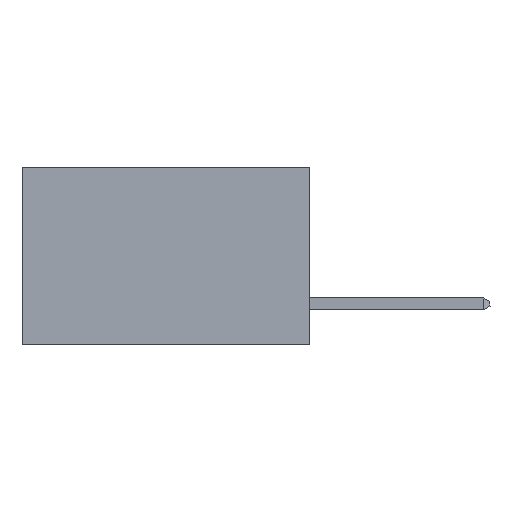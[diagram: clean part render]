
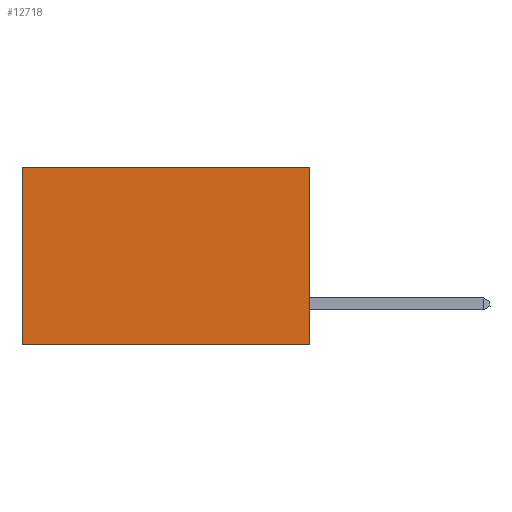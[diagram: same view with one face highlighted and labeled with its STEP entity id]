
A CAD part, left-side view. The second image highlights one B-rep face of the part: STEP entity #12718.
In plain terms, the highlighted planar face has unit normal (-1, 0, 0).
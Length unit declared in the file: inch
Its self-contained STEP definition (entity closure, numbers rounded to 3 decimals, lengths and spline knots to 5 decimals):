
#42 = DIRECTION ( 'NONE',  ( 0., 1., 0. ) ) ;
#250 = LINE ( 'NONE', #8095, #5584 ) ;
#330 = DIRECTION ( 'NONE',  ( 0., 0., -1. ) ) ;
#371 = VERTEX_POINT ( 'NONE', #1072 ) ;
#444 = VECTOR ( 'NONE', #42, 39.37008 ) ;
#823 = LINE ( 'NONE', #10963, #444 ) ;
#824 = DIRECTION ( 'NONE',  ( 1., 0., 0. ) ) ;
#1034 = VECTOR ( 'NONE', #9453, 39.37008 ) ;
#1072 = CARTESIAN_POINT ( 'NONE',  ( 0.2875, 0.6, -0.37 ) ) ;
#1482 = ORIENTED_EDGE ( 'NONE', *, *, #14352, .F. ) ;
#1924 = CARTESIAN_POINT ( 'NONE',  ( 0.2875, 0., 0. ) ) ;
#2628 = AXIS2_PLACEMENT_3D ( 'NONE', #1924, #824, #11736 ) ;
#2763 = CARTESIAN_POINT ( 'NONE',  ( 0.2875, 0., 0. ) ) ;
#3373 = EDGE_CURVE ( 'NONE', #14773, #12495, #250, .T. ) ;
#3547 = LINE ( 'NONE', #10750, #1034 ) ;
#3920 = ORIENTED_EDGE ( 'NONE', *, *, #14530, .F. ) ;
#4230 = CARTESIAN_POINT ( 'NONE',  ( 0.2875, 0., -0.37 ) ) ;
#4263 = VERTEX_POINT ( 'NONE', #4230 ) ;
#4431 = PLANE ( 'NONE',  #2628 ) ;
#5317 = LINE ( 'NONE', #15131, #14573 ) ;
#5584 = VECTOR ( 'NONE', #9321, 39.37008 ) ;
#5759 = CARTESIAN_POINT ( 'NONE',  ( 0.2875, 0.6, 0. ) ) ;
#7109 = ORIENTED_EDGE ( 'NONE', *, *, #3373, .T. ) ;
#8095 = CARTESIAN_POINT ( 'NONE',  ( 0.2875, 0., 0. ) ) ;
#8760 = FACE_OUTER_BOUND ( 'NONE', #9922, .T. ) ;
#9321 = DIRECTION ( 'NONE',  ( 0., 1., 0. ) ) ;
#9453 = DIRECTION ( 'NONE',  ( 0., 0., -1. ) ) ;
#9922 = EDGE_LOOP ( 'NONE', ( #11963, #3920, #1482, #7109 ) ) ;
#10750 = CARTESIAN_POINT ( 'NONE',  ( 0.2875, 0., 0. ) ) ;
#10963 = CARTESIAN_POINT ( 'NONE',  ( 0.2875, 0., -0.37 ) ) ;
#11736 = DIRECTION ( 'NONE',  ( 0., 0., -1. ) ) ;
#11963 = ORIENTED_EDGE ( 'NONE', *, *, #12000, .T. ) ;
#12000 = EDGE_CURVE ( 'NONE', #12495, #371, #5317, .T. ) ;
#12495 = VERTEX_POINT ( 'NONE', #5759 ) ;
#12718 = ADVANCED_FACE ( 'NONE', ( #8760 ), #4431, .F. ) ;
#14352 = EDGE_CURVE ( 'NONE', #14773, #4263, #3547, .T. ) ;
#14530 = EDGE_CURVE ( 'NONE', #4263, #371, #823, .T. ) ;
#14573 = VECTOR ( 'NONE', #330, 39.37008 ) ;
#14773 = VERTEX_POINT ( 'NONE', #2763 ) ;
#15131 = CARTESIAN_POINT ( 'NONE',  ( 0.2875, 0.6, 0. ) ) ;
